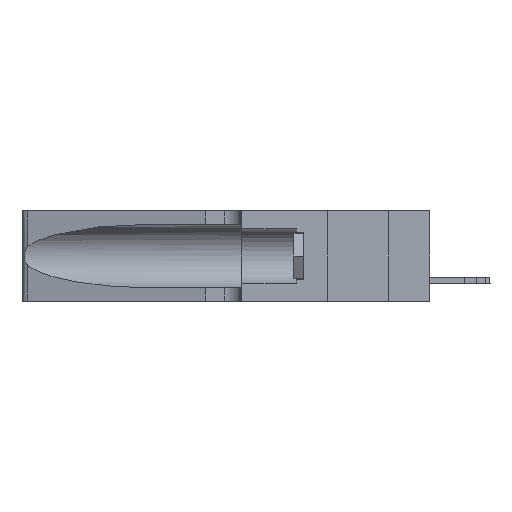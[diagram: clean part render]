
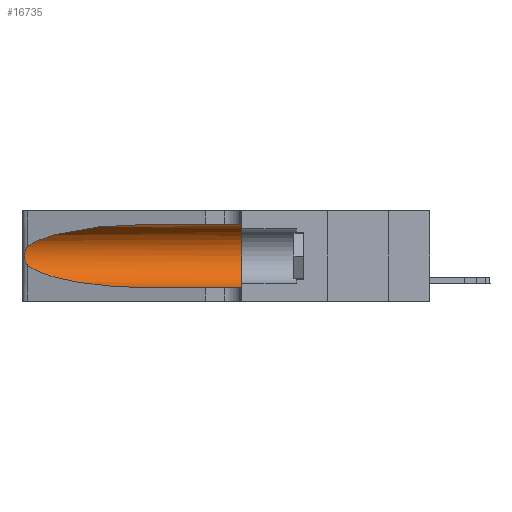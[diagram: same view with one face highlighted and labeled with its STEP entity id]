
A CAD part, left-side view. The second image highlights one B-rep face of the part: STEP entity #16735.
In plain terms, the highlighted cylindrical face has radius 3.308 mm (diameter 6.617 mm), a partial arc.
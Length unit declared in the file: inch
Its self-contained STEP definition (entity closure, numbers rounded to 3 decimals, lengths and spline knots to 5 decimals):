
#826 = CARTESIAN_POINT ( 'NONE',  ( 0.1305, 0.72297, 0.31525 ) ) ;
#955 = ORIENTED_EDGE ( 'NONE', *, *, #16781, .F. ) ;
#1074 = CARTESIAN_POINT ( 'NONE',  ( 0.25639, 1.23186, 0.15144 ) ) ;
#2377 = LINE ( 'NONE', #8449, #31641 ) ;
#2778 = CARTESIAN_POINT ( 'NONE',  ( 0.1305, 0.72297, 0.05475 ) ) ;
#3246 = B_SPLINE_CURVE_WITH_KNOTS ( 'NONE', 3,
 ( #16213, #18852, #31701, #11422, #13880, #26632, #16453, #26746, #31810, #21645, #21527, #1074, #3923, #23949 ),
 .UNSPECIFIED., .F., .F.,
 ( 4, 2, 2, 2, 2, 2, 4 ),
 ( 0., 0.00027, 0.00053, 0.00107, 0.0016, 0.00187, 0.00214 ),
 .UNSPECIFIED. ) ;
#3923 = CARTESIAN_POINT ( 'NONE',  ( 0.25555, 1.22993, 0.14849 ) ) ;
#5667 = CARTESIAN_POINT ( 'NONE',  ( 0.2373, 1.15595, 0.08982 ) ) ;
#7347 = DIRECTION ( 'NONE',  ( 0., 1., 0. ) ) ;
#7818 = DIRECTION ( 'NONE',  ( 0., 0., -1. ) ) ;
#8258 = VERTEX_POINT ( 'NONE', #16226 ) ;
#8449 = CARTESIAN_POINT ( 'NONE',  ( 0.1305, 1.61858, 0.05475 ) ) ;
#8544 = EDGE_CURVE ( 'NONE', #10637, #31466, #28748, .T. ) ;
#8873 = CARTESIAN_POINT ( 'NONE',  ( 0.1305, 0.72297, 0.05475 ) ) ;
#10101 = AXIS2_PLACEMENT_3D ( 'NONE', #19611, #23120, #7818 ) ;
#10637 = VERTEX_POINT ( 'NONE', #22479 ) ;
#10744 = ORIENTED_EDGE ( 'NONE', *, *, #28675, .T. ) ;
#11422 = CARTESIAN_POINT ( 'NONE',  ( 0.25787, 1.23484, 0.2124 ) ) ;
#13880 = CARTESIAN_POINT ( 'NONE',  ( 0.25854, 1.2359, 0.20912 ) ) ;
#13914 = ORIENTED_EDGE ( 'NONE', *, *, #32815, .F. ) ;
#15782 = ORIENTED_EDGE ( 'NONE', *, *, #8544, .T. ) ;
#16213 = CARTESIAN_POINT ( 'NONE',  ( 0.25487, 1.22718, 0.22369 ) ) ;
#16226 = CARTESIAN_POINT ( 'NONE',  ( 0.1305, 0.35, 0.31525 ) ) ;
#16318 = CARTESIAN_POINT ( 'NONE',  ( 0.2373, 1.15595, 0.28018 ) ) ;
#16364 = ORIENTED_EDGE ( 'NONE', *, *, #21990, .T. ) ;
#16453 = CARTESIAN_POINT ( 'NONE',  ( 0.26075, 1.23896, 0.19203 ) ) ;
#16552 = CARTESIAN_POINT ( 'NONE',  ( 0.18966, 0.96281, 0.31525 ) ) ;
#16735 = ADVANCED_FACE ( 'NONE', ( #31581 ), #20059, .F. ) ;
#16781 = EDGE_CURVE ( 'NONE', #8258, #19980, #18352, .T. ) ;
#18352 = CIRCLE ( 'NONE', #24022, 0.13025 ) ;
#18852 = CARTESIAN_POINT ( 'NONE',  ( 0.25555, 1.22994, 0.2215 ) ) ;
#19611 = CARTESIAN_POINT ( 'NONE',  ( 0.1305, 1.61858, 0.185 ) ) ;
#19980 = VERTEX_POINT ( 'NONE', #32112 ) ;
#20059 = CYLINDRICAL_SURFACE ( 'NONE', #10101, 0.13025 ) ;
#20863 = CARTESIAN_POINT ( 'NONE',  ( 0.25487, 1.22718, 0.14631 ) ) ;
#21527 = CARTESIAN_POINT ( 'NONE',  ( 0.25789, 1.23486, 0.15765 ) ) ;
#21645 = CARTESIAN_POINT ( 'NONE',  ( 0.25856, 1.23593, 0.16098 ) ) ;
#21990 = EDGE_CURVE ( 'NONE', #24308, #27857, #29158, .T. ) ;
#22170 = ORIENTED_EDGE ( 'NONE', *, *, #28732, .T. ) ;
#22479 = CARTESIAN_POINT ( 'NONE',  ( 0.1305, 0.72297, 0.31525 ) ) ;
#22748 = CARTESIAN_POINT ( 'NONE',  ( 0.25487, 1.22718, 0.14631 ) ) ;
#22765 = CARTESIAN_POINT ( 'NONE',  ( 0.1305, 0.35, 0.185 ) ) ;
#22807 = CARTESIAN_POINT ( 'NONE',  ( 0.1305, 1.61858, 0.31525 ) ) ;
#23120 = DIRECTION ( 'NONE',  ( 0., -1., 0. ) ) ;
#23949 = CARTESIAN_POINT ( 'NONE',  ( 0.25487, 1.22718, 0.14631 ) ) ;
#24022 = AXIS2_PLACEMENT_3D ( 'NONE', #22765, #7347, #33045 ) ;
#24308 = VERTEX_POINT ( 'NONE', #22748 ) ;
#24732 = CARTESIAN_POINT ( 'NONE',  ( 0.25487, 1.22718, 0.22369 ) ) ;
#24912 = DIRECTION ( 'NONE',  ( 0., -1., 0. ) ) ;
#25086 = CARTESIAN_POINT ( 'NONE',  ( 0.25487, 1.22718, 0.22369 ) ) ;
#25439 = EDGE_LOOP ( 'NONE', ( #15782, #10744, #16364, #22170, #955, #13914 ) ) ;
#25517 = LINE ( 'NONE', #22807, #30749 ) ;
#26308 = CARTESIAN_POINT ( 'NONE',  ( 0.18966, 0.96281, 0.05475 ) ) ;
#26632 = CARTESIAN_POINT ( 'NONE',  ( 0.26018, 1.23835, 0.19895 ) ) ;
#26746 = CARTESIAN_POINT ( 'NONE',  ( 0.26075, 1.23896, 0.178 ) ) ;
#27857 = VERTEX_POINT ( 'NONE', #8873 ) ;
#28675 = EDGE_CURVE ( 'NONE', #31466, #24308, #3246, .T. ) ;
#28732 = EDGE_CURVE ( 'NONE', #27857, #19980, #2377, .T. ) ;
#28748 =( BOUNDED_CURVE ( )  B_SPLINE_CURVE ( 3, ( #826, #16552, #16318, #24732 ),
 .UNSPECIFIED., .F., .T. ) 
 B_SPLINE_CURVE_WITH_KNOTS ( ( 4, 4 ),
 ( 1.5708, 2.84003 ),
 .UNSPECIFIED. ) 
 CURVE ( )  GEOMETRIC_REPRESENTATION_ITEM ( )  RATIONAL_B_SPLINE_CURVE ( ( 1., 0.87, 0.87, 1. ) ) 
 REPRESENTATION_ITEM ( '' )  );
#29158 =( BOUNDED_CURVE ( )  B_SPLINE_CURVE ( 3, ( #20863, #5667, #26308, #2778 ),
 .UNSPECIFIED., .F., .T. ) 
 B_SPLINE_CURVE_WITH_KNOTS ( ( 4, 4 ),
 ( 3.44316, 4.71239 ),
 .UNSPECIFIED. ) 
 CURVE ( )  GEOMETRIC_REPRESENTATION_ITEM ( )  RATIONAL_B_SPLINE_CURVE ( ( 1., 0.87, 0.87, 1. ) ) 
 REPRESENTATION_ITEM ( '' )  );
#29479 = DIRECTION ( 'NONE',  ( 0., -1., 0. ) ) ;
#30749 = VECTOR ( 'NONE', #24912, 39.37008 ) ;
#31466 = VERTEX_POINT ( 'NONE', #25086 ) ;
#31581 = FACE_OUTER_BOUND ( 'NONE', #25439, .T. ) ;
#31641 = VECTOR ( 'NONE', #29479, 39.37008 ) ;
#31701 = CARTESIAN_POINT ( 'NONE',  ( 0.25639, 1.23184, 0.21858 ) ) ;
#31810 = CARTESIAN_POINT ( 'NONE',  ( 0.26017, 1.23833, 0.17102 ) ) ;
#32112 = CARTESIAN_POINT ( 'NONE',  ( 0.1305, 0.35, 0.05475 ) ) ;
#32815 = EDGE_CURVE ( 'NONE', #10637, #8258, #25517, .T. ) ;
#33045 = DIRECTION ( 'NONE',  ( 0., 0., 1. ) ) ;
